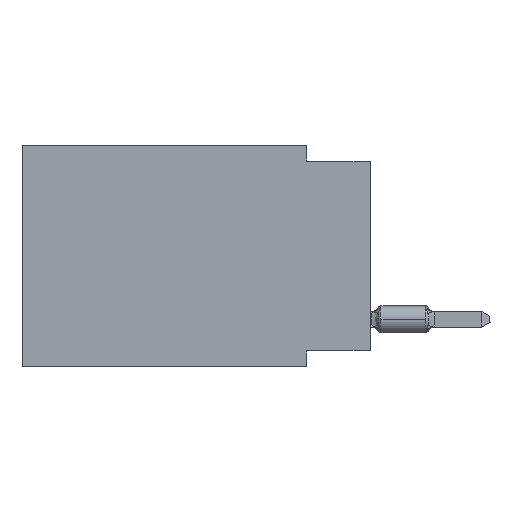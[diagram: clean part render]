
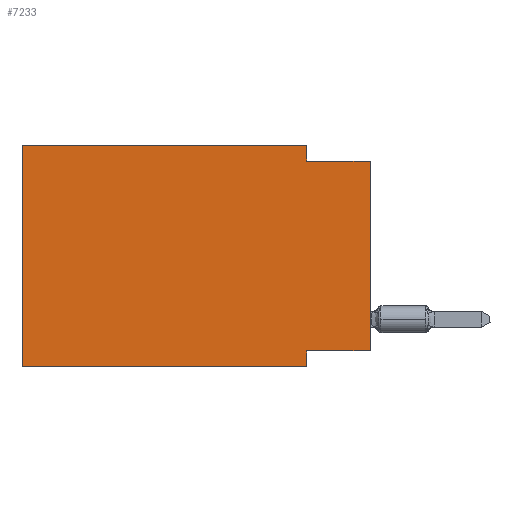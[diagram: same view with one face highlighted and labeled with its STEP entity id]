
A CAD part, left-side view. The second image highlights one B-rep face of the part: STEP entity #7233.
In plain terms, the highlighted planar face has unit normal (-1, 0, 0).
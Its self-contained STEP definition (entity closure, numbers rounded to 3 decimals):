
#38 = VECTOR ( 'NONE', #17193, 1000. ) ;
#590 = EDGE_CURVE ( 'NONE', #18670, #20039, #10820, .T. ) ;
#885 = LINE ( 'NONE', #22727, #13816 ) ;
#2107 = CARTESIAN_POINT ( 'NONE',  ( 0., 13.97, -8.89 ) ) ;
#2215 = ORIENTED_EDGE ( 'NONE', *, *, #32342, .F. ) ;
#2387 = CARTESIAN_POINT ( 'NONE',  ( 0., 13.97, 0. ) ) ;
#3597 = VERTEX_POINT ( 'NONE', #21862 ) ;
#3814 = ORIENTED_EDGE ( 'NONE', *, *, #12249, .F. ) ;
#4685 = EDGE_CURVE ( 'NONE', #6748, #3597, #15391, .T. ) ;
#4791 = VECTOR ( 'NONE', #29859, 1000. ) ;
#5431 = VERTEX_POINT ( 'NONE', #26585 ) ;
#5634 = DIRECTION ( 'NONE',  ( 0., 1., 0. ) ) ;
#5892 = CARTESIAN_POINT ( 'NONE',  ( 0., 0., -0.635 ) ) ;
#6748 = VERTEX_POINT ( 'NONE', #12335 ) ;
#6959 = ORIENTED_EDGE ( 'NONE', *, *, #11432, .T. ) ;
#7233 = ADVANCED_FACE ( 'NONE', ( #14330 ), #23224, .F. ) ;
#7569 = DIRECTION ( 'NONE',  ( 0., 0., -1. ) ) ;
#8547 = CARTESIAN_POINT ( 'NONE',  ( 0., 0., -0.635 ) ) ;
#8897 = CARTESIAN_POINT ( 'NONE',  ( 0., 2.54, -8.255 ) ) ;
#9848 = ORIENTED_EDGE ( 'NONE', *, *, #32801, .F. ) ;
#9989 = CARTESIAN_POINT ( 'NONE',  ( 0., 2.54, -8.89 ) ) ;
#10820 = LINE ( 'NONE', #30469, #35361 ) ;
#10933 = EDGE_LOOP ( 'NONE', ( #30678, #2215, #22676, #9848, #26578, #6959, #3814, #12693 ) ) ;
#11259 = LINE ( 'NONE', #2387, #14812 ) ;
#11432 = EDGE_CURVE ( 'NONE', #5431, #31721, #33217, .T. ) ;
#12249 = EDGE_CURVE ( 'NONE', #20039, #31721, #29809, .T. ) ;
#12335 = CARTESIAN_POINT ( 'NONE',  ( 0., 2.54, 0. ) ) ;
#12693 = ORIENTED_EDGE ( 'NONE', *, *, #590, .F. ) ;
#13816 = VECTOR ( 'NONE', #29012, 1000. ) ;
#14330 = FACE_OUTER_BOUND ( 'NONE', #10933, .T. ) ;
#14812 = VECTOR ( 'NONE', #22557, 1000. ) ;
#14891 = CARTESIAN_POINT ( 'NONE',  ( 0., 13.97, 0. ) ) ;
#15391 = LINE ( 'NONE', #21521, #4791 ) ;
#16942 = DIRECTION ( 'NONE',  ( 1., 0., 0. ) ) ;
#17193 = DIRECTION ( 'NONE',  ( 0., -1., 0. ) ) ;
#18258 = CARTESIAN_POINT ( 'NONE',  ( 0., 13.97, 0. ) ) ;
#18670 = VERTEX_POINT ( 'NONE', #27453 ) ;
#19769 = AXIS2_PLACEMENT_3D ( 'NONE', #14891, #16942, #28237 ) ;
#19811 = LINE ( 'NONE', #5892, #38 ) ;
#20039 = VERTEX_POINT ( 'NONE', #8897 ) ;
#20043 = CARTESIAN_POINT ( 'NONE',  ( 0., 2.54, -8.89 ) ) ;
#21339 = VECTOR ( 'NONE', #7569, 1000. ) ;
#21403 = LINE ( 'NONE', #18258, #34360 ) ;
#21521 = CARTESIAN_POINT ( 'NONE',  ( 0., 2.54, 0. ) ) ;
#21862 = CARTESIAN_POINT ( 'NONE',  ( 0., 2.54, -0.635 ) ) ;
#22007 = VERTEX_POINT ( 'NONE', #8547 ) ;
#22557 = DIRECTION ( 'NONE',  ( 0., 0., 1. ) ) ;
#22676 = ORIENTED_EDGE ( 'NONE', *, *, #4685, .F. ) ;
#22727 = CARTESIAN_POINT ( 'NONE',  ( 0., 0., 0. ) ) ;
#23224 = PLANE ( 'NONE',  #19769 ) ;
#26115 = VERTEX_POINT ( 'NONE', #34557 ) ;
#26578 = ORIENTED_EDGE ( 'NONE', *, *, #29485, .F. ) ;
#26585 = CARTESIAN_POINT ( 'NONE',  ( 0., 13.97, -8.89 ) ) ;
#27453 = CARTESIAN_POINT ( 'NONE',  ( 0., 0., -8.255 ) ) ;
#28237 = DIRECTION ( 'NONE',  ( 0., 0., -1. ) ) ;
#29012 = DIRECTION ( 'NONE',  ( 0., 0., 1. ) ) ;
#29485 = EDGE_CURVE ( 'NONE', #5431, #26115, #11259, .T. ) ;
#29809 = LINE ( 'NONE', #9989, #21339 ) ;
#29859 = DIRECTION ( 'NONE',  ( 0., 0., -1. ) ) ;
#29904 = DIRECTION ( 'NONE',  ( 0., -1., 0. ) ) ;
#30469 = CARTESIAN_POINT ( 'NONE',  ( 0., 0., -8.255 ) ) ;
#30678 = ORIENTED_EDGE ( 'NONE', *, *, #35592, .T. ) ;
#30760 = VECTOR ( 'NONE', #29904, 1000. ) ;
#31721 = VERTEX_POINT ( 'NONE', #20043 ) ;
#32342 = EDGE_CURVE ( 'NONE', #3597, #22007, #19811, .T. ) ;
#32711 = DIRECTION ( 'NONE',  ( 0., -1., 0. ) ) ;
#32801 = EDGE_CURVE ( 'NONE', #26115, #6748, #21403, .T. ) ;
#33217 = LINE ( 'NONE', #2107, #30760 ) ;
#34360 = VECTOR ( 'NONE', #32711, 1000. ) ;
#34557 = CARTESIAN_POINT ( 'NONE',  ( 0., 13.97, 0. ) ) ;
#35361 = VECTOR ( 'NONE', #5634, 1000. ) ;
#35592 = EDGE_CURVE ( 'NONE', #18670, #22007, #885, .T. ) ;
